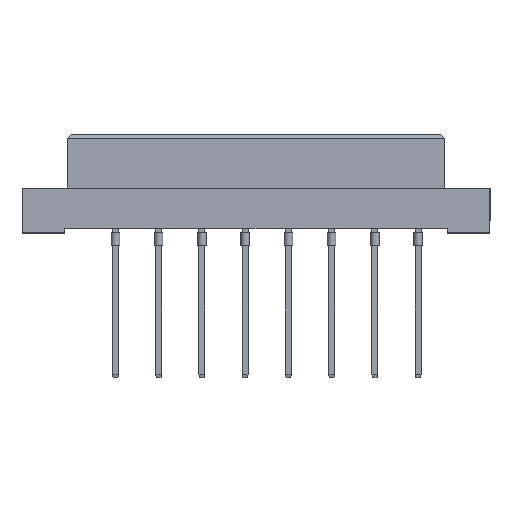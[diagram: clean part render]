
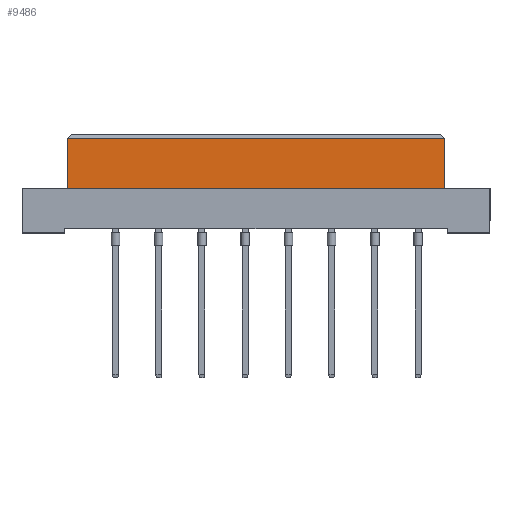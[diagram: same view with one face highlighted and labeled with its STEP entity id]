
A CAD part, top view. The second image highlights one B-rep face of the part: STEP entity #9486.
In plain terms, the highlighted planar face has unit normal (0, 0, 1).
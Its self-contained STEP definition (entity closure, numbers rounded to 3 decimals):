
#141 = EDGE_CURVE ( 'NONE', #17543, #4730, #1783, .T. ) ;
#796 = CARTESIAN_POINT ( 'NONE',  ( -22.2, -6.4, 4.25 ) ) ;
#974 = ORIENTED_EDGE ( 'NONE', *, *, #141, .T. ) ;
#988 = FACE_OUTER_BOUND ( 'NONE', #12841, .T. ) ;
#1476 = CARTESIAN_POINT ( 'NONE',  ( 22.2, -6.4, 4.25 ) ) ;
#1783 = LINE ( 'NONE', #8109, #10952 ) ;
#2286 = AXIS2_PLACEMENT_3D ( 'NONE', #10519, #13422, #10420 ) ;
#2515 = VERTEX_POINT ( 'NONE', #8282 ) ;
#2517 = CARTESIAN_POINT ( 'NONE',  ( 22.2, -6.4, 4.25 ) ) ;
#4584 = LINE ( 'NONE', #1476, #7515 ) ;
#4730 = VERTEX_POINT ( 'NONE', #5123 ) ;
#5123 = CARTESIAN_POINT ( 'NONE',  ( -22.2, -0.5, 4.25 ) ) ;
#5850 = PLANE ( 'NONE',  #2286 ) ;
#6355 = DIRECTION ( 'NONE',  ( -1., 0., 0. ) ) ;
#7185 = DIRECTION ( 'NONE',  ( 1., 0., 0. ) ) ;
#7238 = EDGE_CURVE ( 'NONE', #16506, #4730, #7479, .T. ) ;
#7274 = DIRECTION ( 'NONE',  ( 0., 1., 0. ) ) ;
#7479 = LINE ( 'NONE', #10687, #17802 ) ;
#7515 = VECTOR ( 'NONE', #10704, 1000. ) ;
#8109 = CARTESIAN_POINT ( 'NONE',  ( -22.2, -0.5, 4.25 ) ) ;
#8282 = CARTESIAN_POINT ( 'NONE',  ( 22.2, -6.4, 4.25 ) ) ;
#8305 = ORIENTED_EDGE ( 'NONE', *, *, #7238, .F. ) ;
#9486 = ADVANCED_FACE ( 'NONE', ( #988 ), #5850, .T. ) ;
#10420 = DIRECTION ( 'NONE',  ( 1., 0., 0. ) ) ;
#10519 = CARTESIAN_POINT ( 'NONE',  ( 22.2, -6.4, 4.25 ) ) ;
#10687 = CARTESIAN_POINT ( 'NONE',  ( -22.2, -6.4, 4.25 ) ) ;
#10704 = DIRECTION ( 'NONE',  ( 0., 1., 0. ) ) ;
#10765 = EDGE_CURVE ( 'NONE', #2515, #17543, #4584, .T. ) ;
#10952 = VECTOR ( 'NONE', #6355, 1000. ) ;
#12841 = EDGE_LOOP ( 'NONE', ( #15143, #974, #8305, #15462 ) ) ;
#13368 = CARTESIAN_POINT ( 'NONE',  ( 22.2, -0.5, 4.25 ) ) ;
#13422 = DIRECTION ( 'NONE',  ( 0., 0., 1. ) ) ;
#15143 = ORIENTED_EDGE ( 'NONE', *, *, #10765, .T. ) ;
#15368 = LINE ( 'NONE', #2517, #16048 ) ;
#15462 = ORIENTED_EDGE ( 'NONE', *, *, #18960, .T. ) ;
#16048 = VECTOR ( 'NONE', #7185, 1000. ) ;
#16506 = VERTEX_POINT ( 'NONE', #796 ) ;
#17543 = VERTEX_POINT ( 'NONE', #13368 ) ;
#17802 = VECTOR ( 'NONE', #7274, 1000. ) ;
#18960 = EDGE_CURVE ( 'NONE', #16506, #2515, #15368, .T. ) ;
